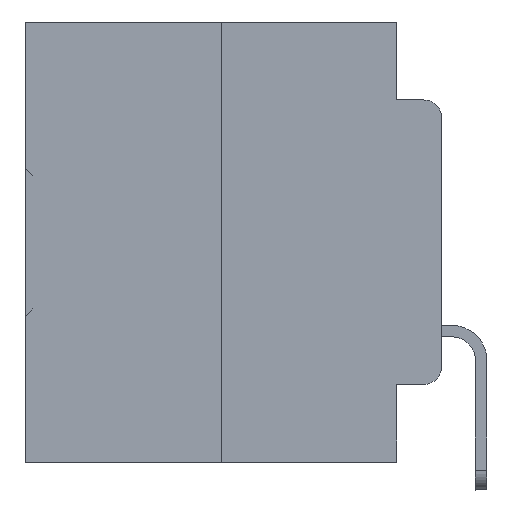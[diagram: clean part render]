
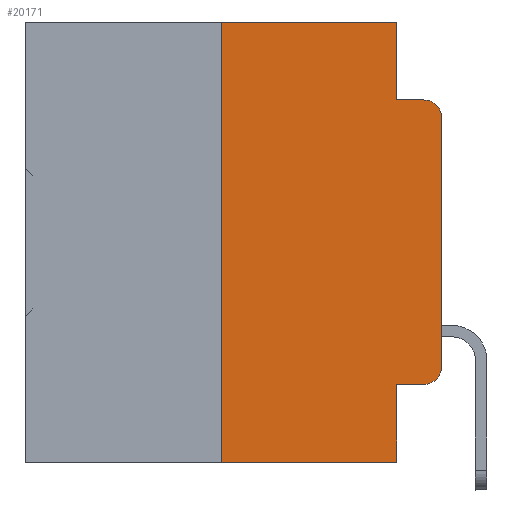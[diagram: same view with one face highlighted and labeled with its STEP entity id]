
A CAD part, left-side view. The second image highlights one B-rep face of the part: STEP entity #20171.
In plain terms, the highlighted planar face has unit normal (-1, 0, 0).
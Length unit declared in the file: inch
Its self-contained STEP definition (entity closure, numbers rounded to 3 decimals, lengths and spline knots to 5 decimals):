
#164 = CARTESIAN_POINT ( 'NONE',  ( 0., 0.02, -0.4115 ) ) ;
#972 = CARTESIAN_POINT ( 'NONE',  ( 0., 0.25, 0. ) ) ;
#2904 = CARTESIAN_POINT ( 'NONE',  ( 0., 0.051, -0.0885 ) ) ;
#3058 = ORIENTED_EDGE ( 'NONE', *, *, #30196, .F. ) ;
#3230 = ORIENTED_EDGE ( 'NONE', *, *, #31532, .T. ) ;
#3439 = CARTESIAN_POINT ( 'NONE',  ( 0., 0.02, -0.0885 ) ) ;
#4756 = PLANE ( 'NONE',  #24984 ) ;
#5006 = EDGE_CURVE ( 'NONE', #27114, #20740, #20945, .T. ) ;
#5174 = DIRECTION ( 'NONE',  ( -1., 0., 0. ) ) ;
#5260 = VECTOR ( 'NONE', #17990, 39.37008 ) ;
#6230 = CARTESIAN_POINT ( 'NONE',  ( 0., 0.051, -0.0885 ) ) ;
#6382 = VECTOR ( 'NONE', #24075, 39.37008 ) ;
#6500 = VECTOR ( 'NONE', #30308, 39.37008 ) ;
#7667 = VERTEX_POINT ( 'NONE', #33209 ) ;
#7753 = CARTESIAN_POINT ( 'NONE',  ( 0., 0.051, 0. ) ) ;
#8567 = EDGE_CURVE ( 'NONE', #35858, #22603, #30775, .T. ) ;
#8859 = VERTEX_POINT ( 'NONE', #6230 ) ;
#8883 = EDGE_CURVE ( 'NONE', #8859, #22603, #28283, .T. ) ;
#8894 = CARTESIAN_POINT ( 'NONE',  ( 0., 0.051, 0. ) ) ;
#12108 = ORIENTED_EDGE ( 'NONE', *, *, #28882, .F. ) ;
#12442 = AXIS2_PLACEMENT_3D ( 'NONE', #13912, #5174, #19265 ) ;
#12451 = EDGE_CURVE ( 'NONE', #18466, #35885, #35053, .T. ) ;
#13122 = DIRECTION ( 'NONE',  ( 1., 0., 0. ) ) ;
#13816 = LINE ( 'NONE', #19709, #6500 ) ;
#13838 = ORIENTED_EDGE ( 'NONE', *, *, #12451, .T. ) ;
#13912 = CARTESIAN_POINT ( 'NONE',  ( 0., 0.02, -0.3915 ) ) ;
#14261 = CARTESIAN_POINT ( 'NONE',  ( 0., 0., -0.1085 ) ) ;
#14838 = ORIENTED_EDGE ( 'NONE', *, *, #18146, .F. ) ;
#15366 = DIRECTION ( 'NONE',  ( 0., 0., -1. ) ) ;
#16076 = FACE_OUTER_BOUND ( 'NONE', #29853, .T. ) ;
#16569 = VERTEX_POINT ( 'NONE', #22346 ) ;
#17990 = DIRECTION ( 'NONE',  ( 0., 0., -1. ) ) ;
#18146 = EDGE_CURVE ( 'NONE', #16569, #27114, #25210, .T. ) ;
#18210 = CARTESIAN_POINT ( 'NONE',  ( 0., 0.051, -0.4115 ) ) ;
#18466 = VERTEX_POINT ( 'NONE', #22170 ) ;
#18891 = DIRECTION ( 'NONE',  ( 0., 0., -1. ) ) ;
#18930 = VECTOR ( 'NONE', #25028, 39.37008 ) ;
#19265 = DIRECTION ( 'NONE',  ( 0., 0., -1. ) ) ;
#19709 = CARTESIAN_POINT ( 'NONE',  ( 0., 0.473, -0.5 ) ) ;
#20171 = ADVANCED_FACE ( 'NONE', ( #16076 ), #4756, .F. ) ;
#20178 = VERTEX_POINT ( 'NONE', #21633 ) ;
#20281 = LINE ( 'NONE', #31767, #28222 ) ;
#20740 = VERTEX_POINT ( 'NONE', #8894 ) ;
#20945 = LINE ( 'NONE', #26863, #6382 ) ;
#21092 = DIRECTION ( 'NONE',  ( -1., 0., 0. ) ) ;
#21633 = CARTESIAN_POINT ( 'NONE',  ( 0., 0., -0.3915 ) ) ;
#22170 = CARTESIAN_POINT ( 'NONE',  ( 0., 0.051, -0.4115 ) ) ;
#22346 = CARTESIAN_POINT ( 'NONE',  ( 0., 0.25, -0.5 ) ) ;
#22479 = CIRCLE ( 'NONE', #12442, 0.02 ) ;
#22603 = VERTEX_POINT ( 'NONE', #3439 ) ;
#23095 = VECTOR ( 'NONE', #25505, 39.37008 ) ;
#23136 = ORIENTED_EDGE ( 'NONE', *, *, #26505, .T. ) ;
#23720 = CARTESIAN_POINT ( 'NONE',  ( 0., 0.051, 0. ) ) ;
#24075 = DIRECTION ( 'NONE',  ( 0., -1., 0. ) ) ;
#24984 = AXIS2_PLACEMENT_3D ( 'NONE', #27364, #13122, #32192 ) ;
#25028 = DIRECTION ( 'NONE',  ( 0., 0., 1. ) ) ;
#25210 = LINE ( 'NONE', #28170, #18930 ) ;
#25505 = DIRECTION ( 'NONE',  ( 0., -1., 0. ) ) ;
#25624 = ORIENTED_EDGE ( 'NONE', *, *, #8567, .T. ) ;
#26292 = ORIENTED_EDGE ( 'NONE', *, *, #8883, .F. ) ;
#26505 = EDGE_CURVE ( 'NONE', #20178, #35858, #20281, .T. ) ;
#26603 = ORIENTED_EDGE ( 'NONE', *, *, #31442, .T. ) ;
#26863 = CARTESIAN_POINT ( 'NONE',  ( 0., 0.473, 0. ) ) ;
#27114 = VERTEX_POINT ( 'NONE', #972 ) ;
#27364 = CARTESIAN_POINT ( 'NONE',  ( 0., 0.473, 0. ) ) ;
#27774 = LINE ( 'NONE', #7753, #35995 ) ;
#28170 = CARTESIAN_POINT ( 'NONE',  ( 0., 0.25, 0. ) ) ;
#28222 = VECTOR ( 'NONE', #28435, 39.37008 ) ;
#28283 = LINE ( 'NONE', #2904, #23095 ) ;
#28435 = DIRECTION ( 'NONE',  ( 0., 0., 1. ) ) ;
#28882 = EDGE_CURVE ( 'NONE', #18466, #7667, #27774, .T. ) ;
#28913 = LINE ( 'NONE', #23720, #5260 ) ;
#29695 = DIRECTION ( 'NONE',  ( 0., -1., 0. ) ) ;
#29853 = EDGE_LOOP ( 'NONE', ( #23136, #25624, #26292, #3058, #35389, #14838, #26603, #12108, #13838, #3230 ) ) ;
#30196 = EDGE_CURVE ( 'NONE', #20740, #8859, #28913, .T. ) ;
#30308 = DIRECTION ( 'NONE',  ( 0., -1., 0. ) ) ;
#30775 = CIRCLE ( 'NONE', #32562, 0.02 ) ;
#31442 = EDGE_CURVE ( 'NONE', #16569, #7667, #13816, .T. ) ;
#31532 = EDGE_CURVE ( 'NONE', #35885, #20178, #22479, .T. ) ;
#31767 = CARTESIAN_POINT ( 'NONE',  ( 0., 0., 0. ) ) ;
#32192 = DIRECTION ( 'NONE',  ( 0., 0., -1. ) ) ;
#32562 = AXIS2_PLACEMENT_3D ( 'NONE', #35326, #21092, #15366 ) ;
#33209 = CARTESIAN_POINT ( 'NONE',  ( 0., 0.051, -0.5 ) ) ;
#35053 = LINE ( 'NONE', #18210, #35610 ) ;
#35326 = CARTESIAN_POINT ( 'NONE',  ( 0., 0.02, -0.1085 ) ) ;
#35389 = ORIENTED_EDGE ( 'NONE', *, *, #5006, .F. ) ;
#35610 = VECTOR ( 'NONE', #29695, 39.37008 ) ;
#35858 = VERTEX_POINT ( 'NONE', #14261 ) ;
#35885 = VERTEX_POINT ( 'NONE', #164 ) ;
#35995 = VECTOR ( 'NONE', #18891, 39.37008 ) ;
